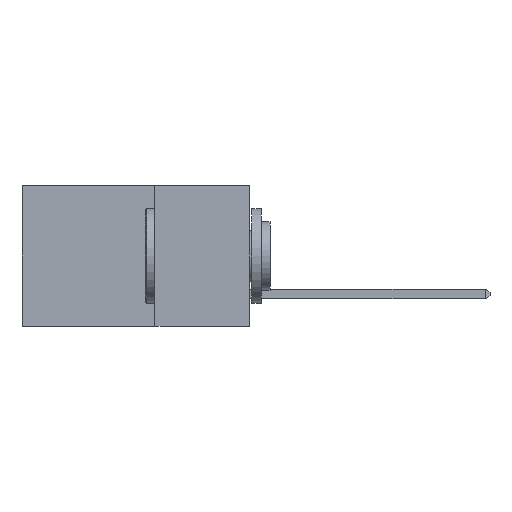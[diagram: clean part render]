
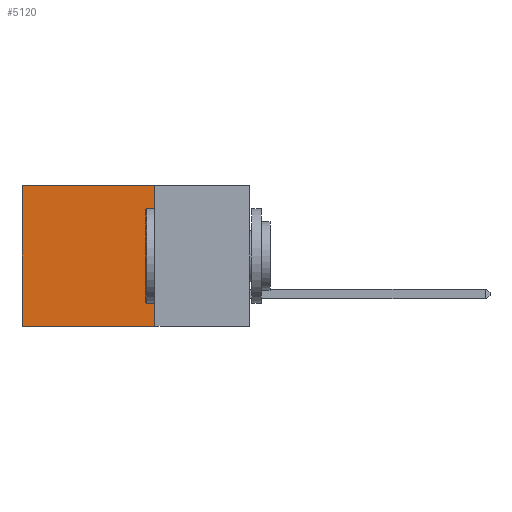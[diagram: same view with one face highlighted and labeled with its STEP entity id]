
A CAD part, left-side view. The second image highlights one B-rep face of the part: STEP entity #5120.
In plain terms, the highlighted planar face has unit normal (-1, 0, 0).
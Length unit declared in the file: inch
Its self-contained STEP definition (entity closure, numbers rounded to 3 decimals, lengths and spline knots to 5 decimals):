
#87 = EDGE_CURVE ( 'NONE', #7221, #6127, #2803, .T. ) ;
#101 = VECTOR ( 'NONE', #8847, 39.37008 ) ;
#1060 = CARTESIAN_POINT ( 'NONE',  ( 0.2875, 0.25, 0. ) ) ;
#1087 = VERTEX_POINT ( 'NONE', #6224 ) ;
#1124 = CARTESIAN_POINT ( 'NONE',  ( 0.2875, 0.25, 0. ) ) ;
#1341 = ORIENTED_EDGE ( 'NONE', *, *, #87, .F. ) ;
#1458 = DIRECTION ( 'NONE',  ( 0., 1., 0. ) ) ;
#2153 = PLANE ( 'NONE',  #4266 ) ;
#2803 = LINE ( 'NONE', #8676, #101 ) ;
#3075 = LINE ( 'NONE', #5817, #5788 ) ;
#3252 = EDGE_CURVE ( 'NONE', #3524, #1087, #3075, .T. ) ;
#3524 = VERTEX_POINT ( 'NONE', #3945 ) ;
#3945 = CARTESIAN_POINT ( 'NONE',  ( 0.2875, 0.6, 0. ) ) ;
#3992 = CARTESIAN_POINT ( 'NONE',  ( 0.2875, 0.25, 0. ) ) ;
#4204 = DIRECTION ( 'NONE',  ( 0., 0., -1. ) ) ;
#4266 = AXIS2_PLACEMENT_3D ( 'NONE', #1124, #10158, #4204 ) ;
#5120 = ADVANCED_FACE ( 'NONE', ( #7135 ), #2153, .F. ) ;
#5788 = VECTOR ( 'NONE', #5886, 39.37008 ) ;
#5817 = CARTESIAN_POINT ( 'NONE',  ( 0.2875, 0.6, 0. ) ) ;
#5886 = DIRECTION ( 'NONE',  ( 0., 0., -1. ) ) ;
#6127 = VERTEX_POINT ( 'NONE', #9801 ) ;
#6224 = CARTESIAN_POINT ( 'NONE',  ( 0.2875, 0.6, -0.37 ) ) ;
#6916 = VECTOR ( 'NONE', #1458, 39.37008 ) ;
#7035 = LINE ( 'NONE', #3992, #11858 ) ;
#7135 = FACE_OUTER_BOUND ( 'NONE', #8195, .T. ) ;
#7221 = VERTEX_POINT ( 'NONE', #1060 ) ;
#7853 = ORIENTED_EDGE ( 'NONE', *, *, #10637, .F. ) ;
#8012 = ORIENTED_EDGE ( 'NONE', *, *, #9726, .T. ) ;
#8195 = EDGE_LOOP ( 'NONE', ( #11599, #7853, #1341, #8012 ) ) ;
#8480 = CARTESIAN_POINT ( 'NONE',  ( 0.2875, 0.25, -0.37 ) ) ;
#8676 = CARTESIAN_POINT ( 'NONE',  ( 0.2875, 0.25, 0. ) ) ;
#8847 = DIRECTION ( 'NONE',  ( 0., 0., -1. ) ) ;
#9726 = EDGE_CURVE ( 'NONE', #7221, #3524, #7035, .T. ) ;
#9801 = CARTESIAN_POINT ( 'NONE',  ( 0.2875, 0.25, -0.37 ) ) ;
#9811 = LINE ( 'NONE', #8480, #6916 ) ;
#10158 = DIRECTION ( 'NONE',  ( 1., 0., 0. ) ) ;
#10637 = EDGE_CURVE ( 'NONE', #6127, #1087, #9811, .T. ) ;
#11599 = ORIENTED_EDGE ( 'NONE', *, *, #3252, .T. ) ;
#11858 = VECTOR ( 'NONE', #11867, 39.37008 ) ;
#11867 = DIRECTION ( 'NONE',  ( 0., 1., 0. ) ) ;
